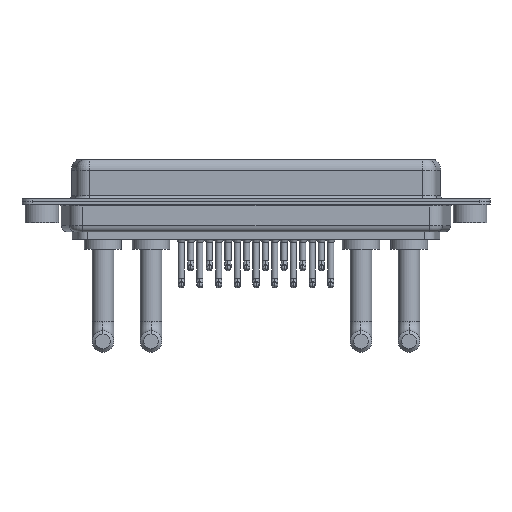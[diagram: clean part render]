
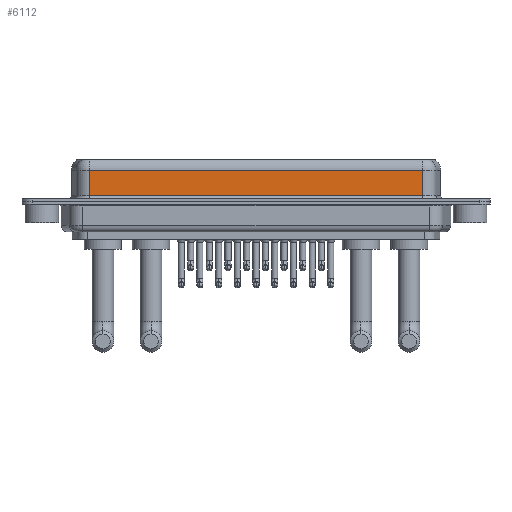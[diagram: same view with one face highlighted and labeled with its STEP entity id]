
A CAD part, front view. The second image highlights one B-rep face of the part: STEP entity #6112.
In plain terms, the highlighted planar face has unit normal (0, -1, 0).
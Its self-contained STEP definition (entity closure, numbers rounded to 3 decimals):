
#252 = LINE ( 'NONE', #9072, #13544 ) ;
#368 = VECTOR ( 'NONE', #7981, 1000. ) ;
#430 = CARTESIAN_POINT ( 'NONE',  ( 56.462, -3.95, 0.9 ) ) ;
#670 = VERTEX_POINT ( 'NONE', #8473 ) ;
#2459 = VECTOR ( 'NONE', #15403, 1000. ) ;
#3212 = VERTEX_POINT ( 'NONE', #430 ) ;
#4508 = AXIS2_PLACEMENT_3D ( 'NONE', #7277, #10968, #14324 ) ;
#4613 = ORIENTED_EDGE ( 'NONE', *, *, #10055, .F. ) ;
#4982 = LINE ( 'NONE', #20381, #8633 ) ;
#5929 = FACE_OUTER_BOUND ( 'NONE', #12862, .T. ) ;
#6112 = ADVANCED_FACE ( 'NONE', ( #5929 ), #9065, .F. ) ;
#7277 = CARTESIAN_POINT ( 'NONE',  ( 56.462, -3.95, 6.4 ) ) ;
#7561 = ORIENTED_EDGE ( 'NONE', *, *, #18446, .T. ) ;
#7607 = EDGE_CURVE ( 'NONE', #670, #3212, #252, .T. ) ;
#7835 = ORIENTED_EDGE ( 'NONE', *, *, #20183, .T. ) ;
#7981 = DIRECTION ( 'NONE',  ( -1., 0., 0. ) ) ;
#8303 = VERTEX_POINT ( 'NONE', #8356 ) ;
#8356 = CARTESIAN_POINT ( 'NONE',  ( 7.038, -3.95, 4.65 ) ) ;
#8473 = CARTESIAN_POINT ( 'NONE',  ( 7.038, -3.95, 0.9 ) ) ;
#8581 = CARTESIAN_POINT ( 'NONE',  ( 7.038, -3.95, 6.4 ) ) ;
#8633 = VECTOR ( 'NONE', #11800, 1000. ) ;
#9065 = PLANE ( 'NONE',  #4508 ) ;
#9072 = CARTESIAN_POINT ( 'NONE',  ( 56.462, -3.95, 0.9 ) ) ;
#10055 = EDGE_CURVE ( 'NONE', #16813, #3212, #4982, .T. ) ;
#10061 = CARTESIAN_POINT ( 'NONE',  ( 56.462, -3.95, 4.65 ) ) ;
#10764 = DIRECTION ( 'NONE',  ( 1., 0., 0. ) ) ;
#10968 = DIRECTION ( 'NONE',  ( 0., 1., 0. ) ) ;
#11800 = DIRECTION ( 'NONE',  ( 0., 0., -1. ) ) ;
#12626 = ORIENTED_EDGE ( 'NONE', *, *, #7607, .T. ) ;
#12862 = EDGE_LOOP ( 'NONE', ( #4613, #7835, #7561, #12626 ) ) ;
#13245 = LINE ( 'NONE', #16480, #368 ) ;
#13544 = VECTOR ( 'NONE', #10764, 1000. ) ;
#13613 = LINE ( 'NONE', #8581, #2459 ) ;
#14324 = DIRECTION ( 'NONE',  ( 0., 0., 1. ) ) ;
#15403 = DIRECTION ( 'NONE',  ( 0., 0., -1. ) ) ;
#16480 = CARTESIAN_POINT ( 'NONE',  ( 56.462, -3.95, 4.65 ) ) ;
#16813 = VERTEX_POINT ( 'NONE', #10061 ) ;
#18446 = EDGE_CURVE ( 'NONE', #8303, #670, #13613, .T. ) ;
#20183 = EDGE_CURVE ( 'NONE', #16813, #8303, #13245, .T. ) ;
#20381 = CARTESIAN_POINT ( 'NONE',  ( 56.462, -3.95, 6.4 ) ) ;
